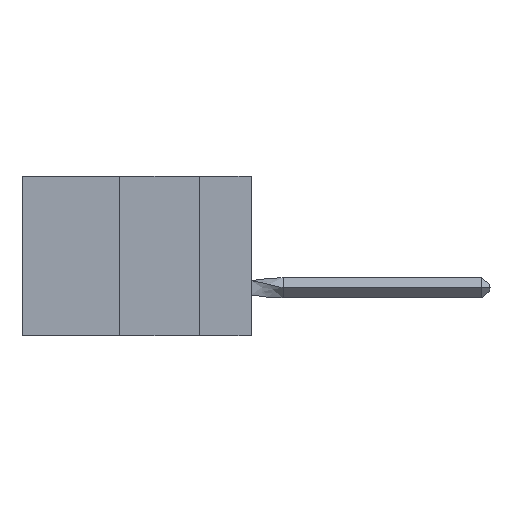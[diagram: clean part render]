
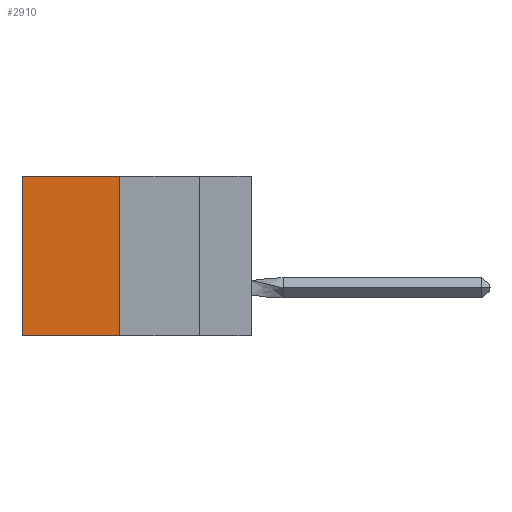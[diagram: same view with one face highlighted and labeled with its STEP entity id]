
A CAD part, left-side view. The second image highlights one B-rep face of the part: STEP entity #2910.
In plain terms, the highlighted planar face has unit normal (-1, 0, 0).
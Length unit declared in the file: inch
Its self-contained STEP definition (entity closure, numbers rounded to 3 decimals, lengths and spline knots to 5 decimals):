
#20 = EDGE_CURVE ( 'NONE', #18682, #28368, #24676, .T. ) ;
#1757 = DIRECTION ( 'NONE',  ( 0., 1., 0. ) ) ;
#2910 = ADVANCED_FACE ( 'NONE', ( #14391 ), #25411, .F. ) ;
#6534 = AXIS2_PLACEMENT_3D ( 'NONE', #10068, #21145, #9684 ) ;
#6676 = EDGE_CURVE ( 'NONE', #8574, #20959, #17801, .T. ) ;
#8016 = CARTESIAN_POINT ( 'NONE',  ( 0.305, 0.72, -0.5 ) ) ;
#8574 = VERTEX_POINT ( 'NONE', #15800 ) ;
#9017 = CARTESIAN_POINT ( 'NONE',  ( 0.305, 0.413, -0.5 ) ) ;
#9684 = DIRECTION ( 'NONE',  ( 0., 0., -1. ) ) ;
#9971 = VECTOR ( 'NONE', #27032, 39.37008 ) ;
#10068 = CARTESIAN_POINT ( 'NONE',  ( 0.305, 0.413, -0.5 ) ) ;
#10571 = ORIENTED_EDGE ( 'NONE', *, *, #19525, .F. ) ;
#12463 = VECTOR ( 'NONE', #19120, 39.37008 ) ;
#14391 = FACE_OUTER_BOUND ( 'NONE', #27563, .T. ) ;
#15187 = CARTESIAN_POINT ( 'NONE',  ( 0.305, 0.72, 0. ) ) ;
#15800 = CARTESIAN_POINT ( 'NONE',  ( 0.305, 0.413, 0. ) ) ;
#16437 = ORIENTED_EDGE ( 'NONE', *, *, #28381, .T. ) ;
#17331 = LINE ( 'NONE', #9017, #9971 ) ;
#17801 = LINE ( 'NONE', #18473, #21982 ) ;
#18473 = CARTESIAN_POINT ( 'NONE',  ( 0.305, 0.413, -0.5 ) ) ;
#18682 = VERTEX_POINT ( 'NONE', #15187 ) ;
#19120 = DIRECTION ( 'NONE',  ( 0., 0., -1. ) ) ;
#19145 = CARTESIAN_POINT ( 'NONE',  ( 0.305, 0.413, -0.5 ) ) ;
#19525 = EDGE_CURVE ( 'NONE', #20959, #28368, #17331, .T. ) ;
#20959 = VERTEX_POINT ( 'NONE', #19145 ) ;
#21145 = DIRECTION ( 'NONE',  ( 1., 0., 0. ) ) ;
#21982 = VECTOR ( 'NONE', #23226, 39.37008 ) ;
#22680 = ORIENTED_EDGE ( 'NONE', *, *, #6676, .F. ) ;
#23226 = DIRECTION ( 'NONE',  ( 0., 0., -1. ) ) ;
#23600 = ORIENTED_EDGE ( 'NONE', *, *, #20, .T. ) ;
#24676 = LINE ( 'NONE', #8016, #12463 ) ;
#25114 = LINE ( 'NONE', #26271, #26521 ) ;
#25411 = PLANE ( 'NONE',  #6534 ) ;
#26271 = CARTESIAN_POINT ( 'NONE',  ( 0.305, 0.413, 0. ) ) ;
#26521 = VECTOR ( 'NONE', #1757, 39.37008 ) ;
#27032 = DIRECTION ( 'NONE',  ( 0., 1., 0. ) ) ;
#27563 = EDGE_LOOP ( 'NONE', ( #23600, #10571, #22680, #16437 ) ) ;
#28368 = VERTEX_POINT ( 'NONE', #28400 ) ;
#28381 = EDGE_CURVE ( 'NONE', #8574, #18682, #25114, .T. ) ;
#28400 = CARTESIAN_POINT ( 'NONE',  ( 0.305, 0.72, -0.5 ) ) ;
